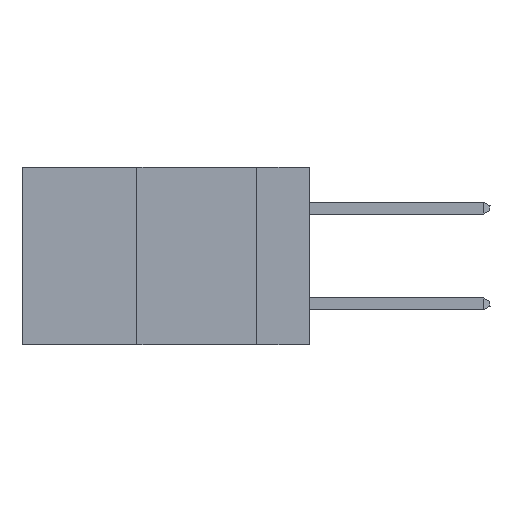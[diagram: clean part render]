
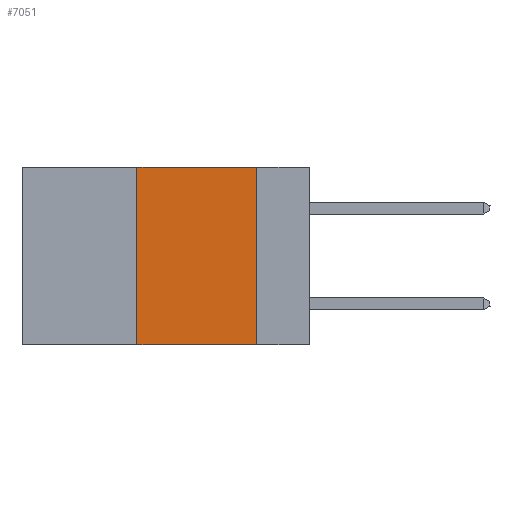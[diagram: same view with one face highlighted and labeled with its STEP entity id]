
A CAD part, left-side view. The second image highlights one B-rep face of the part: STEP entity #7051.
In plain terms, the highlighted planar face has unit normal (-1, 0, 0).
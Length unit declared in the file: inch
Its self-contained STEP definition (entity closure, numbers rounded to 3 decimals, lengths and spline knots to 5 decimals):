
#44 = FACE_OUTER_BOUND ( 'NONE', #12398, .T. ) ;
#625 = DIRECTION ( 'NONE',  ( 0., -1., 0. ) ) ;
#1077 = CARTESIAN_POINT ( 'NONE',  ( 0., 0.36, 0. ) ) ;
#1092 = ORIENTED_EDGE ( 'NONE', *, *, #5469, .F. ) ;
#1335 = VERTEX_POINT ( 'NONE', #5589 ) ;
#1527 = PLANE ( 'NONE',  #14132 ) ;
#2161 = DIRECTION ( 'NONE',  ( 0., 0., -1. ) ) ;
#2211 = ORIENTED_EDGE ( 'NONE', *, *, #17359, .F. ) ;
#2848 = LINE ( 'NONE', #3872, #10489 ) ;
#2910 = VECTOR ( 'NONE', #13136, 39.37008 ) ;
#3254 = DIRECTION ( 'NONE',  ( 1., 0., 0. ) ) ;
#3855 = VERTEX_POINT ( 'NONE', #1077 ) ;
#3872 = CARTESIAN_POINT ( 'NONE',  ( 0., 0.11, 0. ) ) ;
#4684 = CARTESIAN_POINT ( 'NONE',  ( 0., 0.36, 0. ) ) ;
#5469 = EDGE_CURVE ( 'NONE', #1335, #20594, #2848, .T. ) ;
#5584 = VECTOR ( 'NONE', #7960, 39.37008 ) ;
#5589 = CARTESIAN_POINT ( 'NONE',  ( 0., 0.11, 0. ) ) ;
#5689 = CARTESIAN_POINT ( 'NONE',  ( 0., 0.6, -0.37 ) ) ;
#6963 = EDGE_CURVE ( 'NONE', #11032, #3855, #18139, .T. ) ;
#7051 = ADVANCED_FACE ( 'NONE', ( #44 ), #1527, .F. ) ;
#7492 = VECTOR ( 'NONE', #625, 39.37008 ) ;
#7960 = DIRECTION ( 'NONE',  ( 0., 0., 1. ) ) ;
#8625 = ORIENTED_EDGE ( 'NONE', *, *, #9544, .T. ) ;
#9544 = EDGE_CURVE ( 'NONE', #11032, #20594, #15831, .T. ) ;
#10489 = VECTOR ( 'NONE', #2161, 39.37008 ) ;
#11032 = VERTEX_POINT ( 'NONE', #17219 ) ;
#11618 = CARTESIAN_POINT ( 'NONE',  ( 0., 0.6, 0. ) ) ;
#12398 = EDGE_LOOP ( 'NONE', ( #1092, #2211, #20022, #8625 ) ) ;
#12837 = CARTESIAN_POINT ( 'NONE',  ( 0., 0.6, 0. ) ) ;
#13136 = DIRECTION ( 'NONE',  ( 0., -1., 0. ) ) ;
#14132 = AXIS2_PLACEMENT_3D ( 'NONE', #12837, #3254, #14387 ) ;
#14387 = DIRECTION ( 'NONE',  ( 0., 0., -1. ) ) ;
#15625 = LINE ( 'NONE', #11618, #2910 ) ;
#15831 = LINE ( 'NONE', #5689, #7492 ) ;
#17219 = CARTESIAN_POINT ( 'NONE',  ( 0., 0.36, -0.37 ) ) ;
#17359 = EDGE_CURVE ( 'NONE', #3855, #1335, #15625, .T. ) ;
#18139 = LINE ( 'NONE', #4684, #5584 ) ;
#19403 = CARTESIAN_POINT ( 'NONE',  ( 0., 0.11, -0.37 ) ) ;
#20022 = ORIENTED_EDGE ( 'NONE', *, *, #6963, .F. ) ;
#20594 = VERTEX_POINT ( 'NONE', #19403 ) ;
